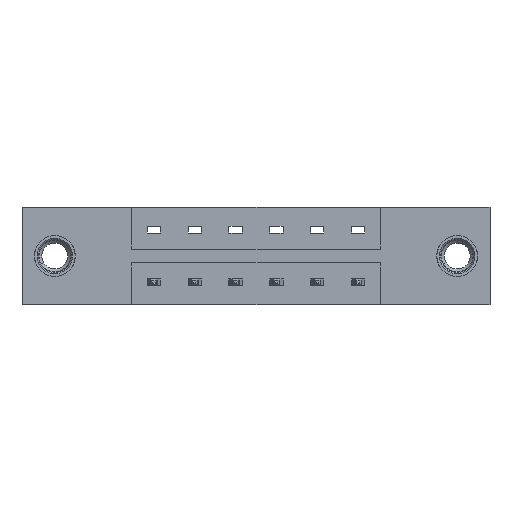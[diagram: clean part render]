
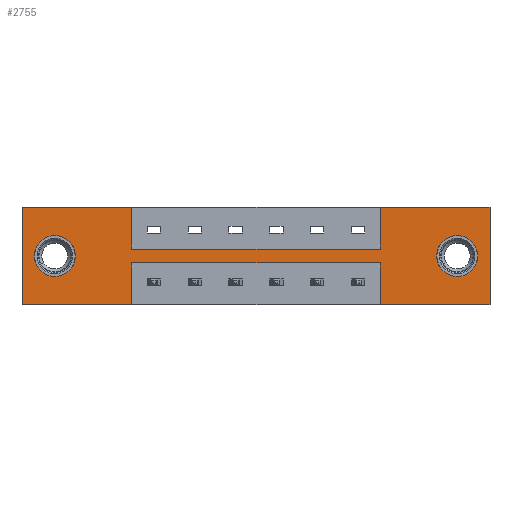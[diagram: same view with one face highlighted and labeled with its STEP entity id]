
A CAD part, front view. The second image highlights one B-rep face of the part: STEP entity #2755.
In plain terms, the highlighted planar face has unit normal (0, -1, 0).
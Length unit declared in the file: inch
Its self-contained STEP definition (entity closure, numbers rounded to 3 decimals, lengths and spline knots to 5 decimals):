
#12 = CARTESIAN_POINT ( 'NONE',  ( 1.3665, 0., -0.2115 ) ) ;
#45 = VECTOR ( 'NONE', #1943, 39.37008 ) ;
#61 = EDGE_CURVE ( 'NONE', #4168, #1601, #2186, .T. ) ;
#63 = VERTEX_POINT ( 'NONE', #371 ) ;
#200 = EDGE_CURVE ( 'NONE', #1522, #4168, #7050, .T. ) ;
#233 = EDGE_LOOP ( 'NONE', ( #757, #3464 ) ) ;
#255 = AXIS2_PLACEMENT_3D ( 'NONE', #4907, #4896, #4892 ) ;
#313 = VECTOR ( 'NONE', #4213, 39.37008 ) ;
#345 = CARTESIAN_POINT ( 'NONE',  ( 1.784, 0., 0. ) ) ;
#371 = CARTESIAN_POINT ( 'NONE',  ( 1.3665, 0., -0.37 ) ) ;
#393 = VERTEX_POINT ( 'NONE', #7751 ) ;
#467 = EDGE_CURVE ( 'NONE', #1601, #4419, #3165, .T. ) ;
#471 = ORIENTED_EDGE ( 'NONE', *, *, #200, .F. ) ;
#563 = VECTOR ( 'NONE', #2641, 39.37008 ) ;
#583 = EDGE_CURVE ( 'NONE', #8020, #1706, #6244, .T. ) ;
#666 = VECTOR ( 'NONE', #8707, 39.37008 ) ;
#698 = EDGE_CURVE ( 'NONE', #4419, #1435, #1667, .T. ) ;
#757 = ORIENTED_EDGE ( 'NONE', *, *, #583, .T. ) ;
#774 = EDGE_CURVE ( 'NONE', #3806, #1522, #3039, .T. ) ;
#995 = FACE_BOUND ( 'NONE', #233, .T. ) ;
#998 = ORIENTED_EDGE ( 'NONE', *, *, #774, .F. ) ;
#1015 = EDGE_CURVE ( 'NONE', #3380, #1818, #4882, .T. ) ;
#1034 = VECTOR ( 'NONE', #5592, 39.37008 ) ;
#1036 = CARTESIAN_POINT ( 'NONE',  ( 0., 0., 0. ) ) ;
#1103 = ORIENTED_EDGE ( 'NONE', *, *, #2446, .T. ) ;
#1149 = ORIENTED_EDGE ( 'NONE', *, *, #1015, .F. ) ;
#1160 = CARTESIAN_POINT ( 'NONE',  ( 0., 0., 0. ) ) ;
#1228 = ORIENTED_EDGE ( 'NONE', *, *, #61, .F. ) ;
#1250 = FACE_BOUND ( 'NONE', #2461, .T. ) ;
#1417 = VECTOR ( 'NONE', #2767, 39.37008 ) ;
#1435 = VERTEX_POINT ( 'NONE', #345 ) ;
#1504 = VERTEX_POINT ( 'NONE', #9435 ) ;
#1522 = VERTEX_POINT ( 'NONE', #9240 ) ;
#1601 = VERTEX_POINT ( 'NONE', #9008 ) ;
#1667 = LINE ( 'NONE', #1160, #1417 ) ;
#1673 = EDGE_LOOP ( 'NONE', ( #3858, #3388, #3357, #2514, #2250, #1228, #471, #998, #4475, #3337, #2721, #1149 ) ) ;
#1706 = VERTEX_POINT ( 'NONE', #8465 ) ;
#1818 = VERTEX_POINT ( 'NONE', #8053 ) ;
#1850 = DIRECTION ( 'NONE',  ( 0., 0., -1. ) ) ;
#1896 = CARTESIAN_POINT ( 'NONE',  ( 0.125, 0., -0.107 ) ) ;
#1943 = DIRECTION ( 'NONE',  ( 1., 0., 0. ) ) ;
#1993 = DIRECTION ( 'NONE',  ( -1., 0., 0. ) ) ;
#2056 = CARTESIAN_POINT ( 'NONE',  ( 0., 0., -0.37 ) ) ;
#2186 = LINE ( 'NONE', #3722, #45 ) ;
#2212 = VECTOR ( 'NONE', #2232, 39.37008 ) ;
#2232 = DIRECTION ( 'NONE',  ( 0., 0., -1. ) ) ;
#2250 = ORIENTED_EDGE ( 'NONE', *, *, #467, .F. ) ;
#2315 = EDGE_CURVE ( 'NONE', #1706, #8020, #6212, .T. ) ;
#2446 = EDGE_CURVE ( 'NONE', #5511, #4527, #5180, .T. ) ;
#2461 = EDGE_LOOP ( 'NONE', ( #1103, #5428 ) ) ;
#2514 = ORIENTED_EDGE ( 'NONE', *, *, #698, .F. ) ;
#2519 = CARTESIAN_POINT ( 'NONE',  ( 0.125, 0., -0.263 ) ) ;
#2641 = DIRECTION ( 'NONE',  ( 0., 0., 1. ) ) ;
#2678 = LINE ( 'NONE', #1036, #563 ) ;
#2721 = ORIENTED_EDGE ( 'NONE', *, *, #9399, .F. ) ;
#2755 = ADVANCED_FACE ( 'NONE', ( #995, #1250, #3117 ), #3227, .T. ) ;
#2767 = DIRECTION ( 'NONE',  ( 1., 0., 0. ) ) ;
#2831 = CARTESIAN_POINT ( 'NONE',  ( 1.784, 0., 0. ) ) ;
#3039 = LINE ( 'NONE', #8580, #666 ) ;
#3116 = DIRECTION ( 'NONE',  ( 0., 0., -1. ) ) ;
#3117 = FACE_OUTER_BOUND ( 'NONE', #1673, .T. ) ;
#3126 = DIRECTION ( 'NONE',  ( 0., -1., 0. ) ) ;
#3165 = LINE ( 'NONE', #5763, #7166 ) ;
#3217 = CARTESIAN_POINT ( 'NONE',  ( 0., 0., -0.37 ) ) ;
#3227 = PLANE ( 'NONE',  #8705 ) ;
#3337 = ORIENTED_EDGE ( 'NONE', *, *, #5496, .F. ) ;
#3357 = ORIENTED_EDGE ( 'NONE', *, *, #5474, .F. ) ;
#3380 = VERTEX_POINT ( 'NONE', #12 ) ;
#3383 = EDGE_CURVE ( 'NONE', #63, #3380, #4167, .T. ) ;
#3388 = ORIENTED_EDGE ( 'NONE', *, *, #4051, .F. ) ;
#3408 = AXIS2_PLACEMENT_3D ( 'NONE', #4277, #4264, #4261 ) ;
#3464 = ORIENTED_EDGE ( 'NONE', *, *, #2315, .T. ) ;
#3570 = VECTOR ( 'NONE', #7060, 39.37008 ) ;
#3578 = CARTESIAN_POINT ( 'NONE',  ( 1.3665, 0., 0. ) ) ;
#3722 = CARTESIAN_POINT ( 'NONE',  ( 0.4175, 0., -0.1585 ) ) ;
#3806 = VERTEX_POINT ( 'NONE', #8965 ) ;
#3822 = VERTEX_POINT ( 'NONE', #8698 ) ;
#3858 = ORIENTED_EDGE ( 'NONE', *, *, #3383, .F. ) ;
#4018 = VECTOR ( 'NONE', #1993, 39.37008 ) ;
#4051 = EDGE_CURVE ( 'NONE', #1504, #63, #5681, .T. ) ;
#4167 = LINE ( 'NONE', #8118, #7226 ) ;
#4168 = VERTEX_POINT ( 'NONE', #6481 ) ;
#4213 = DIRECTION ( 'NONE',  ( 0., 0., -1. ) ) ;
#4251 = LINE ( 'NONE', #2831, #2212 ) ;
#4261 = DIRECTION ( 'NONE',  ( 0., 0., 1. ) ) ;
#4264 = DIRECTION ( 'NONE',  ( 0., 1., 0. ) ) ;
#4277 = CARTESIAN_POINT ( 'NONE',  ( 0.125, 0., -0.185 ) ) ;
#4419 = VERTEX_POINT ( 'NONE', #3578 ) ;
#4475 = ORIENTED_EDGE ( 'NONE', *, *, #9364, .F. ) ;
#4527 = VERTEX_POINT ( 'NONE', #2519 ) ;
#4678 = LINE ( 'NONE', #9135, #313 ) ;
#4882 = LINE ( 'NONE', #6376, #1034 ) ;
#4892 = DIRECTION ( 'NONE',  ( 0., 0., 1. ) ) ;
#4896 = DIRECTION ( 'NONE',  ( 0., 1., 0. ) ) ;
#4907 = CARTESIAN_POINT ( 'NONE',  ( 0.125, 0., -0.185 ) ) ;
#5180 = CIRCLE ( 'NONE', #255, 0.078 ) ;
#5217 = VECTOR ( 'NONE', #1850, 39.37008 ) ;
#5298 = EDGE_CURVE ( 'NONE', #4527, #5511, #5772, .T. ) ;
#5428 = ORIENTED_EDGE ( 'NONE', *, *, #5298, .T. ) ;
#5464 = DIRECTION ( 'NONE',  ( 0., 0., -1. ) ) ;
#5472 = DIRECTION ( 'NONE',  ( 0., 1., 0. ) ) ;
#5474 = EDGE_CURVE ( 'NONE', #1435, #1504, #4251, .T. ) ;
#5480 = CARTESIAN_POINT ( 'NONE',  ( 1.659, 0., -0.185 ) ) ;
#5496 = EDGE_CURVE ( 'NONE', #3822, #393, #7769, .T. ) ;
#5511 = VERTEX_POINT ( 'NONE', #1896 ) ;
#5592 = DIRECTION ( 'NONE',  ( -1., 0., 0. ) ) ;
#5681 = LINE ( 'NONE', #7181, #3570 ) ;
#5763 = CARTESIAN_POINT ( 'NONE',  ( 1.3665, 0., -0.1585 ) ) ;
#5772 = CIRCLE ( 'NONE', #3408, 0.078 ) ;
#5794 = DIRECTION ( 'NONE',  ( 0., 0., 1. ) ) ;
#5899 = CARTESIAN_POINT ( 'NONE',  ( 1.659, 0., -0.107 ) ) ;
#5930 = AXIS2_PLACEMENT_3D ( 'NONE', #7380, #7052, #6771 ) ;
#6212 = CIRCLE ( 'NONE', #7421, 0.078 ) ;
#6244 = CIRCLE ( 'NONE', #5930, 0.078 ) ;
#6376 = CARTESIAN_POINT ( 'NONE',  ( 0.4175, 0., -0.2115 ) ) ;
#6481 = CARTESIAN_POINT ( 'NONE',  ( 0.4175, 0., -0.1585 ) ) ;
#6771 = DIRECTION ( 'NONE',  ( 0., 0., -1. ) ) ;
#7050 = LINE ( 'NONE', #7937, #5217 ) ;
#7052 = DIRECTION ( 'NONE',  ( 0., 1., 0. ) ) ;
#7060 = DIRECTION ( 'NONE',  ( -1., 0., 0. ) ) ;
#7166 = VECTOR ( 'NONE', #5794, 39.37008 ) ;
#7181 = CARTESIAN_POINT ( 'NONE',  ( 0., 0., -0.37 ) ) ;
#7226 = VECTOR ( 'NONE', #8269, 39.37008 ) ;
#7380 = CARTESIAN_POINT ( 'NONE',  ( 1.659, 0., -0.185 ) ) ;
#7421 = AXIS2_PLACEMENT_3D ( 'NONE', #5480, #5472, #5464 ) ;
#7751 = CARTESIAN_POINT ( 'NONE',  ( 0., 0., -0.37 ) ) ;
#7769 = LINE ( 'NONE', #2056, #4018 ) ;
#7937 = CARTESIAN_POINT ( 'NONE',  ( 0.4175, 0., -0.1585 ) ) ;
#8020 = VERTEX_POINT ( 'NONE', #5899 ) ;
#8053 = CARTESIAN_POINT ( 'NONE',  ( 0.4175, 0., -0.2115 ) ) ;
#8118 = CARTESIAN_POINT ( 'NONE',  ( 1.3665, 0., -0.2115 ) ) ;
#8269 = DIRECTION ( 'NONE',  ( 0., 0., 1. ) ) ;
#8465 = CARTESIAN_POINT ( 'NONE',  ( 1.659, 0., -0.263 ) ) ;
#8580 = CARTESIAN_POINT ( 'NONE',  ( 0., 0., 0. ) ) ;
#8698 = CARTESIAN_POINT ( 'NONE',  ( 0.4175, 0., -0.37 ) ) ;
#8705 = AXIS2_PLACEMENT_3D ( 'NONE', #3217, #3126, #3116 ) ;
#8707 = DIRECTION ( 'NONE',  ( 1., 0., 0. ) ) ;
#8965 = CARTESIAN_POINT ( 'NONE',  ( 0., 0., 0. ) ) ;
#9008 = CARTESIAN_POINT ( 'NONE',  ( 1.3665, 0., -0.1585 ) ) ;
#9135 = CARTESIAN_POINT ( 'NONE',  ( 0.4175, 0., -0.2115 ) ) ;
#9240 = CARTESIAN_POINT ( 'NONE',  ( 0.4175, 0., 0. ) ) ;
#9364 = EDGE_CURVE ( 'NONE', #393, #3806, #2678, .T. ) ;
#9399 = EDGE_CURVE ( 'NONE', #1818, #3822, #4678, .T. ) ;
#9435 = CARTESIAN_POINT ( 'NONE',  ( 1.784, 0., -0.37 ) ) ;
